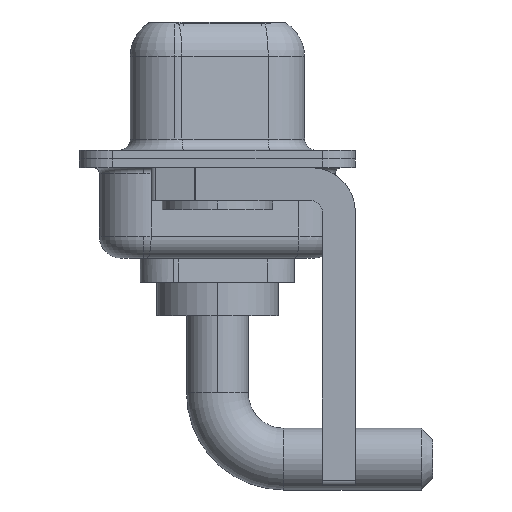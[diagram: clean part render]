
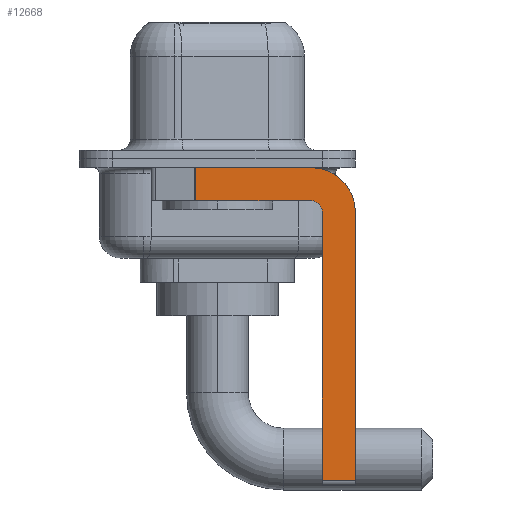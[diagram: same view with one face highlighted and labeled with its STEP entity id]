
A CAD part, left-side view. The second image highlights one B-rep face of the part: STEP entity #12668.
In plain terms, the highlighted planar face has unit normal (-1, 0, 0).
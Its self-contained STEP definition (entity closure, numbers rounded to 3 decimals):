
#89 = VECTOR ( 'NONE', #12895, 1000. ) ;
#464 = CARTESIAN_POINT ( 'NONE',  ( -2.9, -4.75, -2.4 ) ) ;
#520 = DIRECTION ( 'NONE',  ( 0., 1., 0. ) ) ;
#534 = ORIENTED_EDGE ( 'NONE', *, *, #11626, .F. ) ;
#1056 = CARTESIAN_POINT ( 'NONE',  ( -2.9, -6.25, -2.4 ) ) ;
#1194 = AXIS2_PLACEMENT_3D ( 'NONE', #6901, #10833, #9863 ) ;
#1277 = ORIENTED_EDGE ( 'NONE', *, *, #4220, .T. ) ;
#2274 = LINE ( 'NONE', #10672, #6783 ) ;
#2394 = DIRECTION ( 'NONE',  ( 0., 0., 1. ) ) ;
#3040 = LINE ( 'NONE', #11027, #3915 ) ;
#3289 = VERTEX_POINT ( 'NONE', #8804 ) ;
#3363 = VERTEX_POINT ( 'NONE', #12293 ) ;
#3516 = EDGE_LOOP ( 'NONE', ( #3529, #1277, #9076, #3703, #534, #8574, #4572, #7005 ) ) ;
#3529 = ORIENTED_EDGE ( 'NONE', *, *, #5276, .F. ) ;
#3613 = LINE ( 'NONE', #12715, #8280 ) ;
#3703 = ORIENTED_EDGE ( 'NONE', *, *, #7778, .F. ) ;
#3870 = EDGE_CURVE ( 'NONE', #8981, #3289, #3040, .T. ) ;
#3915 = VECTOR ( 'NONE', #10489, 1000. ) ;
#4220 = EDGE_CURVE ( 'NONE', #8133, #8763, #3613, .T. ) ;
#4293 = VECTOR ( 'NONE', #520, 1000. ) ;
#4297 = CARTESIAN_POINT ( 'NONE',  ( -2.9, 0.978, -0.4 ) ) ;
#4572 = ORIENTED_EDGE ( 'NONE', *, *, #3870, .F. ) ;
#4681 = CARTESIAN_POINT ( 'NONE',  ( -2.9, -4.25, -2.4 ) ) ;
#5276 = EDGE_CURVE ( 'NONE', #8133, #10117, #8585, .T. ) ;
#6476 = DIRECTION ( 'NONE',  ( 0., 0., 1. ) ) ;
#6783 = VECTOR ( 'NONE', #2394, 1000. ) ;
#6901 = CARTESIAN_POINT ( 'NONE',  ( -2.9, -4.25, -2.4 ) ) ;
#7005 = ORIENTED_EDGE ( 'NONE', *, *, #8594, .F. ) ;
#7162 = CARTESIAN_POINT ( 'NONE',  ( -2.9, -4.25, -0.4 ) ) ;
#7205 = CIRCLE ( 'NONE', #8650, 2. ) ;
#7419 = DIRECTION ( 'NONE',  ( 0., -1., 0. ) ) ;
#7577 = DIRECTION ( 'NONE',  ( -1., 0., 0. ) ) ;
#7601 = DIRECTION ( 'NONE',  ( 0., 0., -1. ) ) ;
#7681 = VERTEX_POINT ( 'NONE', #10279 ) ;
#7692 = FACE_OUTER_BOUND ( 'NONE', #3516, .T. ) ;
#7778 = EDGE_CURVE ( 'NONE', #9098, #7681, #9933, .T. ) ;
#7880 = EDGE_CURVE ( 'NONE', #7681, #8763, #12493, .T. ) ;
#7883 = PLANE ( 'NONE',  #1194 ) ;
#8133 = VERTEX_POINT ( 'NONE', #4297 ) ;
#8280 = VECTOR ( 'NONE', #7601, 1000. ) ;
#8574 = ORIENTED_EDGE ( 'NONE', *, *, #9045, .T. ) ;
#8585 = LINE ( 'NONE', #10616, #12511 ) ;
#8594 = EDGE_CURVE ( 'NONE', #10117, #8981, #7205, .T. ) ;
#8650 = AXIS2_PLACEMENT_3D ( 'NONE', #9495, #9437, #11209 ) ;
#8678 = CARTESIAN_POINT ( 'NONE',  ( -2.9, -4.25, -1.9 ) ) ;
#8763 = VERTEX_POINT ( 'NONE', #12635 ) ;
#8804 = CARTESIAN_POINT ( 'NONE',  ( -2.9, -6.25, -14.55 ) ) ;
#8888 = CARTESIAN_POINT ( 'NONE',  ( -2.9, -4.25, -14.55 ) ) ;
#8981 = VERTEX_POINT ( 'NONE', #1056 ) ;
#9045 = EDGE_CURVE ( 'NONE', #3363, #3289, #10076, .T. ) ;
#9076 = ORIENTED_EDGE ( 'NONE', *, *, #7880, .F. ) ;
#9098 = VERTEX_POINT ( 'NONE', #464 ) ;
#9437 = DIRECTION ( 'NONE',  ( 1., 0., 0. ) ) ;
#9495 = CARTESIAN_POINT ( 'NONE',  ( -2.9, -4.25, -2.4 ) ) ;
#9863 = DIRECTION ( 'NONE',  ( 0., 0., -1. ) ) ;
#9933 = CIRCLE ( 'NONE', #10144, 0.5 ) ;
#10076 = LINE ( 'NONE', #8888, #89 ) ;
#10117 = VERTEX_POINT ( 'NONE', #7162 ) ;
#10144 = AXIS2_PLACEMENT_3D ( 'NONE', #4681, #7577, #6476 ) ;
#10279 = CARTESIAN_POINT ( 'NONE',  ( -2.9, -4.25, -1.9 ) ) ;
#10489 = DIRECTION ( 'NONE',  ( 0., 0., -1. ) ) ;
#10616 = CARTESIAN_POINT ( 'NONE',  ( -2.9, 3., -0.4 ) ) ;
#10672 = CARTESIAN_POINT ( 'NONE',  ( -2.9, -4.75, -14.8 ) ) ;
#10833 = DIRECTION ( 'NONE',  ( 1., 0., 0. ) ) ;
#11027 = CARTESIAN_POINT ( 'NONE',  ( -2.9, -6.25, -2.4 ) ) ;
#11209 = DIRECTION ( 'NONE',  ( 0., 0., -1. ) ) ;
#11626 = EDGE_CURVE ( 'NONE', #3363, #9098, #2274, .T. ) ;
#12293 = CARTESIAN_POINT ( 'NONE',  ( -2.9, -4.75, -14.55 ) ) ;
#12493 = LINE ( 'NONE', #8678, #4293 ) ;
#12511 = VECTOR ( 'NONE', #7419, 1000. ) ;
#12635 = CARTESIAN_POINT ( 'NONE',  ( -2.9, 0.978, -1.9 ) ) ;
#12668 = ADVANCED_FACE ( 'NONE', ( #7692 ), #7883, .F. ) ;
#12715 = CARTESIAN_POINT ( 'NONE',  ( -2.9, 0.978, -1.9 ) ) ;
#12895 = DIRECTION ( 'NONE',  ( 0., -1., 0. ) ) ;
